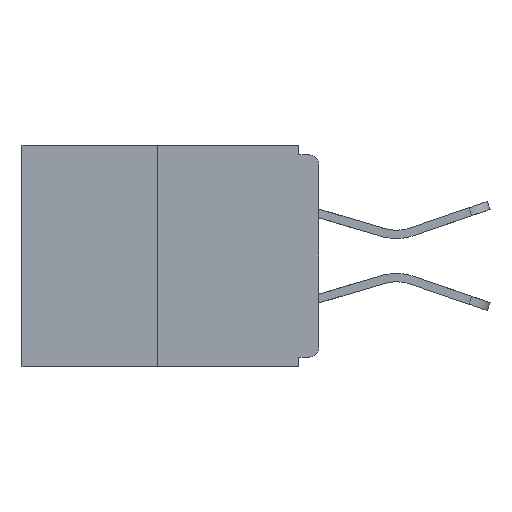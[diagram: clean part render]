
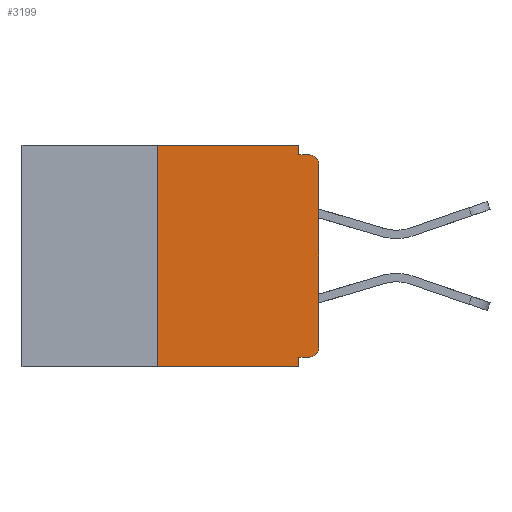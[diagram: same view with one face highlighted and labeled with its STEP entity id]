
A CAD part, left-side view. The second image highlights one B-rep face of the part: STEP entity #3199.
In plain terms, the highlighted planar face has unit normal (-1, 0, 0).
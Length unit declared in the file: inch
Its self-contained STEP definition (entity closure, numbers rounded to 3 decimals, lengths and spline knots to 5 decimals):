
#20 = ORIENTED_EDGE ( 'NONE', *, *, #20211, .F. ) ;
#93 = CARTESIAN_POINT ( 'NONE',  ( 0., 0.25, -0.343 ) ) ;
#413 = EDGE_CURVE ( 'NONE', #15151, #24144, #8522, .T. ) ;
#533 = DIRECTION ( 'NONE',  ( 0., -1., 0. ) ) ;
#1022 = CARTESIAN_POINT ( 'NONE',  ( 0., 0.46, -0.343 ) ) ;
#1275 = VECTOR ( 'NONE', #20049, 39.37008 ) ;
#2784 = ORIENTED_EDGE ( 'NONE', *, *, #19408, .F. ) ;
#2813 = CARTESIAN_POINT ( 'NONE',  ( 0., 0.46, 0. ) ) ;
#2904 = VECTOR ( 'NONE', #533, 39.37008 ) ;
#2964 = EDGE_CURVE ( 'NONE', #17971, #4849, #10004, .T. ) ;
#3199 = ADVANCED_FACE ( 'NONE', ( #15554 ), #14641, .F. ) ;
#3434 = VECTOR ( 'NONE', #10271, 39.37008 ) ;
#3555 = CARTESIAN_POINT ( 'NONE',  ( 0., 0., 0. ) ) ;
#3625 = ORIENTED_EDGE ( 'NONE', *, *, #21850, .T. ) ;
#4062 = CARTESIAN_POINT ( 'NONE',  ( 0., 0., -0.015 ) ) ;
#4119 = DIRECTION ( 'NONE',  ( -1., 0., 0. ) ) ;
#4237 = VECTOR ( 'NONE', #15978, 39.37008 ) ;
#4528 = VECTOR ( 'NONE', #15664, 39.37008 ) ;
#4635 = VERTEX_POINT ( 'NONE', #18708 ) ;
#4849 = VERTEX_POINT ( 'NONE', #21903 ) ;
#4980 = VERTEX_POINT ( 'NONE', #5492 ) ;
#5016 = AXIS2_PLACEMENT_3D ( 'NONE', #6174, #4119, #24777 ) ;
#5492 = CARTESIAN_POINT ( 'NONE',  ( 0., 0.031, -0.328 ) ) ;
#5564 = EDGE_CURVE ( 'NONE', #18316, #24144, #11483, .T. ) ;
#5772 = ORIENTED_EDGE ( 'NONE', *, *, #7977, .F. ) ;
#6160 = LINE ( 'NONE', #24494, #1275 ) ;
#6174 = CARTESIAN_POINT ( 'NONE',  ( 0., 0.015, -0.03 ) ) ;
#6225 = AXIS2_PLACEMENT_3D ( 'NONE', #9097, #8539, #17570 ) ;
#6472 = ORIENTED_EDGE ( 'NONE', *, *, #21718, .T. ) ;
#7565 = VECTOR ( 'NONE', #14571, 39.37008 ) ;
#7977 = EDGE_CURVE ( 'NONE', #19570, #4980, #6160, .T. ) ;
#8393 = LINE ( 'NONE', #2813, #2904 ) ;
#8522 = LINE ( 'NONE', #4062, #20254 ) ;
#8539 = DIRECTION ( 'NONE',  ( -1., 0., 0. ) ) ;
#9097 = CARTESIAN_POINT ( 'NONE',  ( 0., 0.015, -0.313 ) ) ;
#9144 = ORIENTED_EDGE ( 'NONE', *, *, #5564, .T. ) ;
#10004 = LINE ( 'NONE', #1022, #4528 ) ;
#10271 = DIRECTION ( 'NONE',  ( 0., 0., -1. ) ) ;
#11483 = CIRCLE ( 'NONE', #5016, 0.015 ) ;
#12090 = LINE ( 'NONE', #16411, #7565 ) ;
#12329 = VECTOR ( 'NONE', #18074, 39.37008 ) ;
#12522 = CARTESIAN_POINT ( 'NONE',  ( 0., 0.46, 0. ) ) ;
#12995 = LINE ( 'NONE', #3555, #12329 ) ;
#13694 = ORIENTED_EDGE ( 'NONE', *, *, #413, .F. ) ;
#13782 = CARTESIAN_POINT ( 'NONE',  ( 0., 0.25, 0. ) ) ;
#13846 = CARTESIAN_POINT ( 'NONE',  ( 0., 0., -0.03 ) ) ;
#14292 = CIRCLE ( 'NONE', #6225, 0.015 ) ;
#14466 = LINE ( 'NONE', #23049, #3434 ) ;
#14540 = EDGE_CURVE ( 'NONE', #17734, #21287, #8393, .T. ) ;
#14571 = DIRECTION ( 'NONE',  ( 0., 0., -1. ) ) ;
#14641 = PLANE ( 'NONE',  #24606 ) ;
#15151 = VERTEX_POINT ( 'NONE', #23722 ) ;
#15554 = FACE_OUTER_BOUND ( 'NONE', #18666, .T. ) ;
#15664 = DIRECTION ( 'NONE',  ( 0., -1., 0. ) ) ;
#15978 = DIRECTION ( 'NONE',  ( 0., 0., 1. ) ) ;
#16411 = CARTESIAN_POINT ( 'NONE',  ( 0., 0.031, -0.343 ) ) ;
#17570 = DIRECTION ( 'NONE',  ( 0., 0., -1. ) ) ;
#17734 = VERTEX_POINT ( 'NONE', #24314 ) ;
#17812 = ORIENTED_EDGE ( 'NONE', *, *, #14540, .F. ) ;
#17971 = VERTEX_POINT ( 'NONE', #93 ) ;
#18074 = DIRECTION ( 'NONE',  ( 0., 0., 1. ) ) ;
#18316 = VERTEX_POINT ( 'NONE', #13846 ) ;
#18497 = DIRECTION ( 'NONE',  ( 0., -1., 0. ) ) ;
#18666 = EDGE_LOOP ( 'NONE', ( #17812, #26770, #21610, #20, #5772, #3625, #6472, #9144, #13694, #2784 ) ) ;
#18708 = CARTESIAN_POINT ( 'NONE',  ( 0., 0., -0.313 ) ) ;
#18941 = CARTESIAN_POINT ( 'NONE',  ( 0., 0.015, -0.015 ) ) ;
#19408 = EDGE_CURVE ( 'NONE', #21287, #15151, #14466, .T. ) ;
#19570 = VERTEX_POINT ( 'NONE', #20600 ) ;
#20049 = DIRECTION ( 'NONE',  ( 0., 1., 0. ) ) ;
#20211 = EDGE_CURVE ( 'NONE', #4980, #4849, #12090, .T. ) ;
#20254 = VECTOR ( 'NONE', #18497, 39.37008 ) ;
#20600 = CARTESIAN_POINT ( 'NONE',  ( 0., 0.015, -0.328 ) ) ;
#21287 = VERTEX_POINT ( 'NONE', #26682 ) ;
#21610 = ORIENTED_EDGE ( 'NONE', *, *, #2964, .T. ) ;
#21718 = EDGE_CURVE ( 'NONE', #4635, #18316, #12995, .T. ) ;
#21840 = EDGE_CURVE ( 'NONE', #17971, #17734, #22736, .T. ) ;
#21850 = EDGE_CURVE ( 'NONE', #19570, #4635, #14292, .T. ) ;
#21903 = CARTESIAN_POINT ( 'NONE',  ( 0., 0.031, -0.343 ) ) ;
#22736 = LINE ( 'NONE', #13782, #4237 ) ;
#23049 = CARTESIAN_POINT ( 'NONE',  ( 0., 0.031, 0. ) ) ;
#23722 = CARTESIAN_POINT ( 'NONE',  ( 0., 0.031, -0.015 ) ) ;
#24144 = VERTEX_POINT ( 'NONE', #18941 ) ;
#24314 = CARTESIAN_POINT ( 'NONE',  ( 0., 0.25, 0. ) ) ;
#24494 = CARTESIAN_POINT ( 'NONE',  ( 0., 0., -0.328 ) ) ;
#24606 = AXIS2_PLACEMENT_3D ( 'NONE', #12522, #26690, #24625 ) ;
#24625 = DIRECTION ( 'NONE',  ( 0., 0., -1. ) ) ;
#24777 = DIRECTION ( 'NONE',  ( 0., 0., -1. ) ) ;
#26682 = CARTESIAN_POINT ( 'NONE',  ( 0., 0.031, 0. ) ) ;
#26690 = DIRECTION ( 'NONE',  ( 1., 0., 0. ) ) ;
#26770 = ORIENTED_EDGE ( 'NONE', *, *, #21840, .F. ) ;
